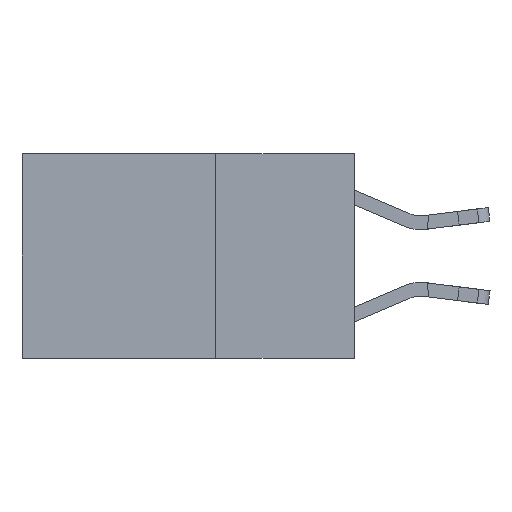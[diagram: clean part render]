
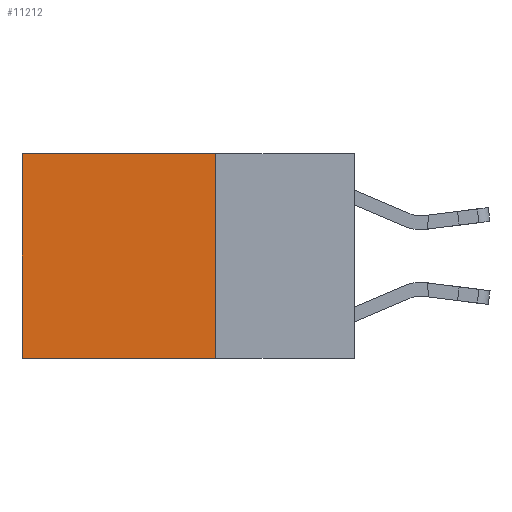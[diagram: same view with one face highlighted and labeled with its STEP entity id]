
A CAD part, left-side view. The second image highlights one B-rep face of the part: STEP entity #11212.
In plain terms, the highlighted planar face has unit normal (-1, 0, 0).
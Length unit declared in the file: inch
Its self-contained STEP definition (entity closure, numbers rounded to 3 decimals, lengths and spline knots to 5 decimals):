
#330 = DIRECTION ( 'NONE',  ( 0., 1., 0. ) ) ;
#600 = CARTESIAN_POINT ( 'NONE',  ( 0.2625, 0.25, 0. ) ) ;
#1964 = CARTESIAN_POINT ( 'NONE',  ( 0.2625, 0.25, 0. ) ) ;
#1974 = DIRECTION ( 'NONE',  ( 0., 0., -1. ) ) ;
#2112 = FACE_OUTER_BOUND ( 'NONE', #6798, .T. ) ;
#2470 = CARTESIAN_POINT ( 'NONE',  ( 0.2625, 0.6, -0.37 ) ) ;
#2658 = LINE ( 'NONE', #1964, #7844 ) ;
#2728 = DIRECTION ( 'NONE',  ( 0., 0., -1. ) ) ;
#2967 = EDGE_CURVE ( 'NONE', #5892, #8714, #2658, .T. ) ;
#3187 = EDGE_CURVE ( 'NONE', #5892, #11866, #10403, .T. ) ;
#3452 = ORIENTED_EDGE ( 'NONE', *, *, #8096, .F. ) ;
#3794 = VECTOR ( 'NONE', #4454, 39.37008 ) ;
#4334 = LINE ( 'NONE', #6659, #11547 ) ;
#4454 = DIRECTION ( 'NONE',  ( 0., 1., 0. ) ) ;
#4851 = ORIENTED_EDGE ( 'NONE', *, *, #3187, .T. ) ;
#4996 = DIRECTION ( 'NONE',  ( 0., 0., -1. ) ) ;
#5448 = CARTESIAN_POINT ( 'NONE',  ( 0.2625, 0.25, -0.37 ) ) ;
#5541 = CARTESIAN_POINT ( 'NONE',  ( 0.2625, 0.25, 0. ) ) ;
#5892 = VERTEX_POINT ( 'NONE', #5541 ) ;
#6478 = LINE ( 'NONE', #5448, #3794 ) ;
#6659 = CARTESIAN_POINT ( 'NONE',  ( 0.2625, 0.6, 0. ) ) ;
#6798 = EDGE_LOOP ( 'NONE', ( #8628, #3452, #8148, #4851 ) ) ;
#6948 = PLANE ( 'NONE',  #7335 ) ;
#7335 = AXIS2_PLACEMENT_3D ( 'NONE', #7836, #10634, #4996 ) ;
#7836 = CARTESIAN_POINT ( 'NONE',  ( 0.2625, 0.25, 0. ) ) ;
#7844 = VECTOR ( 'NONE', #1974, 39.37008 ) ;
#7981 = VECTOR ( 'NONE', #330, 39.37008 ) ;
#8096 = EDGE_CURVE ( 'NONE', #8714, #9161, #6478, .T. ) ;
#8148 = ORIENTED_EDGE ( 'NONE', *, *, #2967, .F. ) ;
#8628 = ORIENTED_EDGE ( 'NONE', *, *, #10991, .T. ) ;
#8714 = VERTEX_POINT ( 'NONE', #9496 ) ;
#9161 = VERTEX_POINT ( 'NONE', #2470 ) ;
#9496 = CARTESIAN_POINT ( 'NONE',  ( 0.2625, 0.25, -0.37 ) ) ;
#10403 = LINE ( 'NONE', #600, #7981 ) ;
#10634 = DIRECTION ( 'NONE',  ( 1., 0., 0. ) ) ;
#10991 = EDGE_CURVE ( 'NONE', #11866, #9161, #4334, .T. ) ;
#11212 = ADVANCED_FACE ( 'NONE', ( #2112 ), #6948, .F. ) ;
#11312 = CARTESIAN_POINT ( 'NONE',  ( 0.2625, 0.6, 0. ) ) ;
#11547 = VECTOR ( 'NONE', #2728, 39.37008 ) ;
#11866 = VERTEX_POINT ( 'NONE', #11312 ) ;
